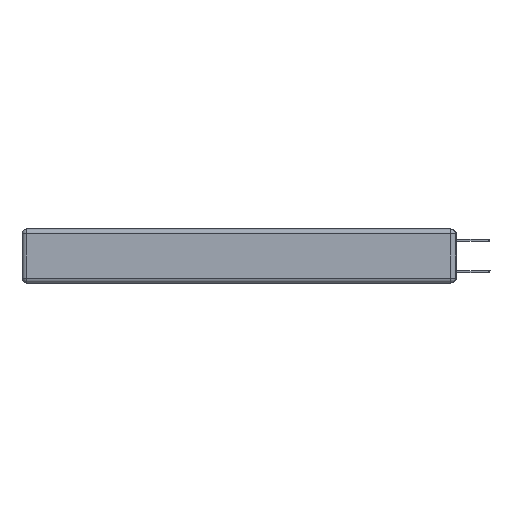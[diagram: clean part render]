
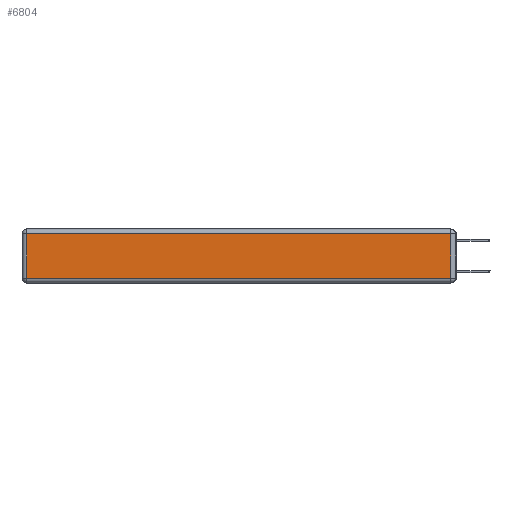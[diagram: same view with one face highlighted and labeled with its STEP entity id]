
A CAD part, left-side view. The second image highlights one B-rep face of the part: STEP entity #6804.
In plain terms, the highlighted planar face has unit normal (-1, 0, 0).
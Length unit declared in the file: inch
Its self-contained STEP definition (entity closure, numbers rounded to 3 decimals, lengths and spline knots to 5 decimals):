
#73 = CARTESIAN_POINT ( 'NONE',  ( 0., 2.72, -0.313 ) ) ;
#603 = VERTEX_POINT ( 'NONE', #15986 ) ;
#1907 = EDGE_CURVE ( 'NONE', #4437, #603, #11181, .T. ) ;
#2763 = VECTOR ( 'NONE', #20422, 39.37008 ) ;
#2951 = CARTESIAN_POINT ( 'NONE',  ( 0., 2.72, -0.343 ) ) ;
#3138 = VERTEX_POINT ( 'NONE', #9946 ) ;
#3250 = ORIENTED_EDGE ( 'NONE', *, *, #4531, .T. ) ;
#3293 = VECTOR ( 'NONE', #8698, 39.37008 ) ;
#3332 = VECTOR ( 'NONE', #10864, 39.37008 ) ;
#3723 = CARTESIAN_POINT ( 'NONE',  ( 0., 2.75, -0.03 ) ) ;
#4437 = VERTEX_POINT ( 'NONE', #73 ) ;
#4531 = EDGE_CURVE ( 'NONE', #7772, #3138, #21771, .T. ) ;
#6804 = ADVANCED_FACE ( 'NONE', ( #22216 ), #8897, .T. ) ;
#7164 = LINE ( 'NONE', #2951, #19095 ) ;
#7772 = VERTEX_POINT ( 'NONE', #19101 ) ;
#8698 = DIRECTION ( 'NONE',  ( 0., -1., 0. ) ) ;
#8897 = PLANE ( 'NONE',  #11618 ) ;
#9756 = CARTESIAN_POINT ( 'NONE',  ( 0., 0.03, -0.343 ) ) ;
#9946 = CARTESIAN_POINT ( 'NONE',  ( 0., 2.72, -0.03 ) ) ;
#10864 = DIRECTION ( 'NONE',  ( 0., 1., 0. ) ) ;
#11181 = LINE ( 'NONE', #18619, #3293 ) ;
#11618 = AXIS2_PLACEMENT_3D ( 'NONE', #16711, #12128, #20025 ) ;
#11885 = ORIENTED_EDGE ( 'NONE', *, *, #16555, .T. ) ;
#12022 = LINE ( 'NONE', #9756, #2763 ) ;
#12128 = DIRECTION ( 'NONE',  ( -1., 0., 0. ) ) ;
#14054 = EDGE_CURVE ( 'NONE', #3138, #4437, #7164, .T. ) ;
#14282 = EDGE_LOOP ( 'NONE', ( #15054, #11885, #3250, #15956 ) ) ;
#15054 = ORIENTED_EDGE ( 'NONE', *, *, #1907, .T. ) ;
#15152 = DIRECTION ( 'NONE',  ( 0., 0., -1. ) ) ;
#15956 = ORIENTED_EDGE ( 'NONE', *, *, #14054, .T. ) ;
#15986 = CARTESIAN_POINT ( 'NONE',  ( 0., 0.03, -0.313 ) ) ;
#16555 = EDGE_CURVE ( 'NONE', #603, #7772, #12022, .T. ) ;
#16711 = CARTESIAN_POINT ( 'NONE',  ( 0., 0., -0.343 ) ) ;
#18619 = CARTESIAN_POINT ( 'NONE',  ( 0., 0., -0.313 ) ) ;
#19095 = VECTOR ( 'NONE', #15152, 39.37008 ) ;
#19101 = CARTESIAN_POINT ( 'NONE',  ( 0., 0.03, -0.03 ) ) ;
#20025 = DIRECTION ( 'NONE',  ( 0., 0., 1. ) ) ;
#20422 = DIRECTION ( 'NONE',  ( 0., 0., 1. ) ) ;
#21771 = LINE ( 'NONE', #3723, #3332 ) ;
#22216 = FACE_OUTER_BOUND ( 'NONE', #14282, .T. ) ;
